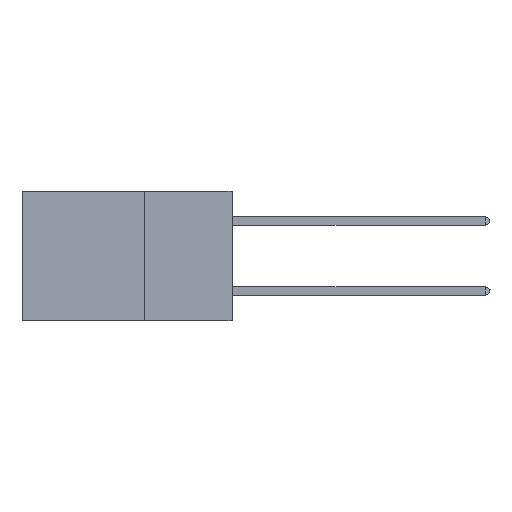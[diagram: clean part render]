
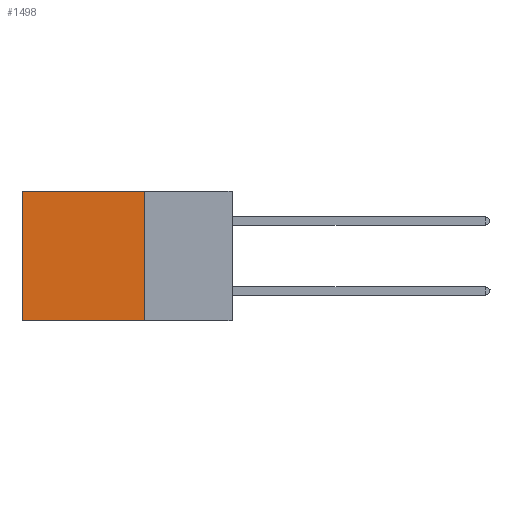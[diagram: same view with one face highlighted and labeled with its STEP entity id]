
A CAD part, left-side view. The second image highlights one B-rep face of the part: STEP entity #1498.
In plain terms, the highlighted planar face has unit normal (-1, 0, 0).
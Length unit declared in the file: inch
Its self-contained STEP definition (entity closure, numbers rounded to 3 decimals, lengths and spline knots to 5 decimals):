
#302 = VERTEX_POINT ( 'NONE', #39175 ) ;
#1038 = VECTOR ( 'NONE', #34855, 39.37008 ) ;
#1162 = ORIENTED_EDGE ( 'NONE', *, *, #31176, .T. ) ;
#1278 = VERTEX_POINT ( 'NONE', #31017 ) ;
#1498 = ADVANCED_FACE ( 'NONE', ( #12205 ), #22992, .F. ) ;
#1695 = VERTEX_POINT ( 'NONE', #27259 ) ;
#1727 = DIRECTION ( 'NONE',  ( 0., 1., 0. ) ) ;
#3376 = CARTESIAN_POINT ( 'NONE',  ( 0.2875, 0.25, 0. ) ) ;
#3620 = AXIS2_PLACEMENT_3D ( 'NONE', #3376, #23121, #13538 ) ;
#5322 = CARTESIAN_POINT ( 'NONE',  ( 0.2875, 0.25, 0. ) ) ;
#6256 = ORIENTED_EDGE ( 'NONE', *, *, #21877, .T. ) ;
#8621 = CARTESIAN_POINT ( 'NONE',  ( 0.2875, 0.6, 0. ) ) ;
#10779 = VECTOR ( 'NONE', #21915, 39.37008 ) ;
#12205 = FACE_OUTER_BOUND ( 'NONE', #25057, .T. ) ;
#13538 = DIRECTION ( 'NONE',  ( 0., 0., -1. ) ) ;
#13657 = CARTESIAN_POINT ( 'NONE',  ( 0.2875, 0.6, -0.37 ) ) ;
#15551 = EDGE_CURVE ( 'NONE', #1278, #16426, #16931, .T. ) ;
#16426 = VERTEX_POINT ( 'NONE', #13657 ) ;
#16931 = LINE ( 'NONE', #34569, #34365 ) ;
#17417 = LINE ( 'NONE', #33937, #36907 ) ;
#18462 = LINE ( 'NONE', #8621, #10779 ) ;
#21877 = EDGE_CURVE ( 'NONE', #302, #1695, #23071, .T. ) ;
#21915 = DIRECTION ( 'NONE',  ( 0., 0., -1. ) ) ;
#22992 = PLANE ( 'NONE',  #3620 ) ;
#23071 = LINE ( 'NONE', #5322, #1038 ) ;
#23121 = DIRECTION ( 'NONE',  ( 1., 0., 0. ) ) ;
#25057 = EDGE_LOOP ( 'NONE', ( #1162, #26674, #34956, #6256 ) ) ;
#26674 = ORIENTED_EDGE ( 'NONE', *, *, #15551, .F. ) ;
#27162 = DIRECTION ( 'NONE',  ( 0., 0., -1. ) ) ;
#27259 = CARTESIAN_POINT ( 'NONE',  ( 0.2875, 0.6, 0. ) ) ;
#31017 = CARTESIAN_POINT ( 'NONE',  ( 0.2875, 0.25, -0.37 ) ) ;
#31176 = EDGE_CURVE ( 'NONE', #1695, #16426, #18462, .T. ) ;
#31546 = EDGE_CURVE ( 'NONE', #302, #1278, #17417, .T. ) ;
#33937 = CARTESIAN_POINT ( 'NONE',  ( 0.2875, 0.25, 0. ) ) ;
#34365 = VECTOR ( 'NONE', #1727, 39.37008 ) ;
#34569 = CARTESIAN_POINT ( 'NONE',  ( 0.2875, 0.25, -0.37 ) ) ;
#34855 = DIRECTION ( 'NONE',  ( 0., 1., 0. ) ) ;
#34956 = ORIENTED_EDGE ( 'NONE', *, *, #31546, .F. ) ;
#36907 = VECTOR ( 'NONE', #27162, 39.37008 ) ;
#39175 = CARTESIAN_POINT ( 'NONE',  ( 0.2875, 0.25, 0. ) ) ;
